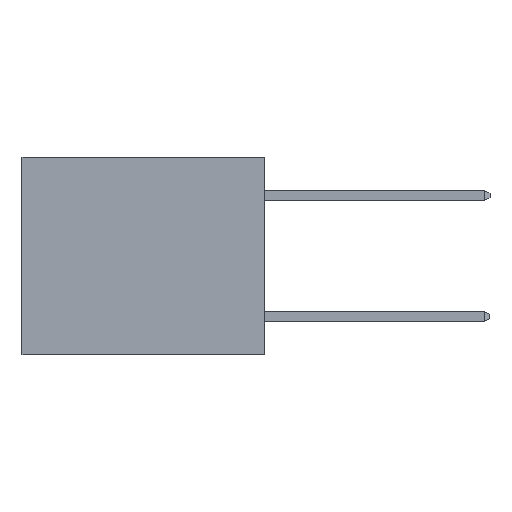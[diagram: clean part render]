
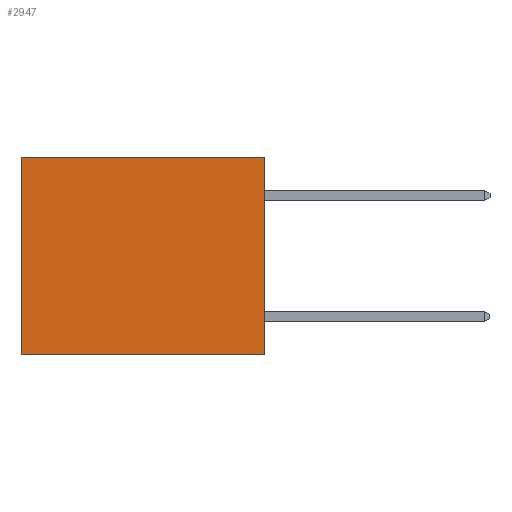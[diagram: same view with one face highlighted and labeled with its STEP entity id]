
A CAD part, left-side view. The second image highlights one B-rep face of the part: STEP entity #2947.
In plain terms, the highlighted planar face has unit normal (-1, 0, 0).
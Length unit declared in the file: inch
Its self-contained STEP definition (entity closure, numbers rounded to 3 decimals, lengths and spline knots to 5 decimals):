
#58 = DIRECTION ( 'NONE',  ( 0., 0., -1. ) ) ;
#382 = EDGE_CURVE ( 'NONE', #11560, #9487, #2731, .T. ) ;
#504 = CARTESIAN_POINT ( 'NONE',  ( 0.3165, 0., -0.49 ) ) ;
#1046 = EDGE_CURVE ( 'NONE', #1849, #11560, #3436, .T. ) ;
#1482 = ORIENTED_EDGE ( 'NONE', *, *, #1046, .F. ) ;
#1606 = ORIENTED_EDGE ( 'NONE', *, *, #11792, .T. ) ;
#1777 = CARTESIAN_POINT ( 'NONE',  ( 0.3165, 0., -0.49 ) ) ;
#1849 = VERTEX_POINT ( 'NONE', #5908 ) ;
#2009 = VECTOR ( 'NONE', #58, 39.37008 ) ;
#2448 = CARTESIAN_POINT ( 'NONE',  ( 0.3165, 0.6, 0. ) ) ;
#2731 = LINE ( 'NONE', #1777, #10071 ) ;
#2947 = ADVANCED_FACE ( 'NONE', ( #3833 ), #6942, .F. ) ;
#3436 = LINE ( 'NONE', #8491, #6876 ) ;
#3703 = VERTEX_POINT ( 'NONE', #2448 ) ;
#3833 = FACE_OUTER_BOUND ( 'NONE', #11246, .T. ) ;
#4689 = ORIENTED_EDGE ( 'NONE', *, *, #5217, .T. ) ;
#5217 = EDGE_CURVE ( 'NONE', #1849, #3703, #7183, .T. ) ;
#5280 = LINE ( 'NONE', #8265, #2009 ) ;
#5439 = ORIENTED_EDGE ( 'NONE', *, *, #382, .F. ) ;
#5549 = DIRECTION ( 'NONE',  ( 0., 1., 0. ) ) ;
#5908 = CARTESIAN_POINT ( 'NONE',  ( 0.3165, 0., 0. ) ) ;
#6653 = AXIS2_PLACEMENT_3D ( 'NONE', #504, #6894, #7785 ) ;
#6876 = VECTOR ( 'NONE', #9538, 39.37008 ) ;
#6894 = DIRECTION ( 'NONE',  ( 1., 0., 0. ) ) ;
#6942 = PLANE ( 'NONE',  #6653 ) ;
#7183 = LINE ( 'NONE', #9857, #10605 ) ;
#7785 = DIRECTION ( 'NONE',  ( 0., 0., -1. ) ) ;
#7877 = CARTESIAN_POINT ( 'NONE',  ( 0.3165, 0., -0.49 ) ) ;
#8265 = CARTESIAN_POINT ( 'NONE',  ( 0.3165, 0.6, -0.49 ) ) ;
#8282 = CARTESIAN_POINT ( 'NONE',  ( 0.3165, 0.6, -0.49 ) ) ;
#8491 = CARTESIAN_POINT ( 'NONE',  ( 0.3165, 0., -0.49 ) ) ;
#9024 = DIRECTION ( 'NONE',  ( 0., 1., 0. ) ) ;
#9487 = VERTEX_POINT ( 'NONE', #8282 ) ;
#9538 = DIRECTION ( 'NONE',  ( 0., 0., -1. ) ) ;
#9857 = CARTESIAN_POINT ( 'NONE',  ( 0.3165, 0., 0. ) ) ;
#10071 = VECTOR ( 'NONE', #5549, 39.37008 ) ;
#10605 = VECTOR ( 'NONE', #9024, 39.37008 ) ;
#11246 = EDGE_LOOP ( 'NONE', ( #1606, #5439, #1482, #4689 ) ) ;
#11560 = VERTEX_POINT ( 'NONE', #7877 ) ;
#11792 = EDGE_CURVE ( 'NONE', #3703, #9487, #5280, .T. ) ;
